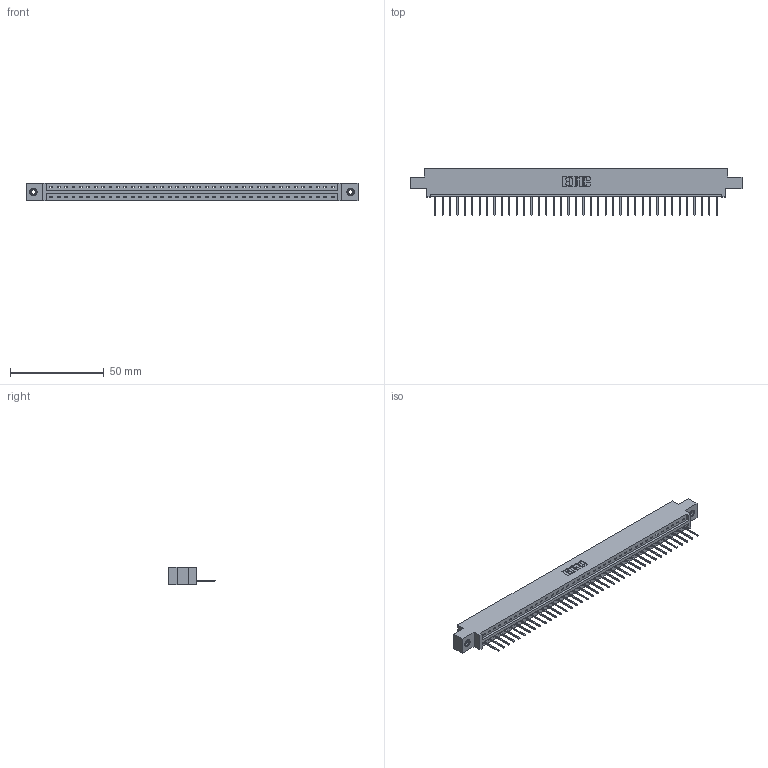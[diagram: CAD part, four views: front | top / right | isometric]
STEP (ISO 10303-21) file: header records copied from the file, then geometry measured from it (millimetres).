
FILE_DESCRIPTION (( 'STEP AP203' ), '1' );
FILE_NAME ('387-039-523-608.STEP', '2019-10-04T17:11:48', ( '' ), ( '' ), 'SwSTEP 2.0', 'SolidWorks 2016', '' );
FILE_SCHEMA (( 'CONFIG_CONTROL_DESIGN' ));
Length unit declared in the file: inch
Products named in the file (4): 337 Part_0.170 Offset - 0.156 Dia-TI; 345-250-001_345-250-003-102; 387-039-523-608; 345-292-001_345-293-123
Assembly tree (42 placements, depth 2):
  387-039-523-608
    337 Part_0.170 Offset - 0.156 Dia-TI
    345-292-001_345-293-123  x39
    345-250-001_345-250-003-102  x2
Bounding box: 177.55 x 25.15 x 9.4 mm (x, y, z)
Volume: 18276.3 mm3; surface area: 19029.7 mm2
Topology: 42 solids, 42 shells, 2596 faces, 7791 edges, 5134 vertices
Faces by surface type: plane 1900, cylinder 680, cone 12, torus 4
Entity records: 30714 total; most frequent: CARTESIAN_POINT 5330, ORIENTED_EDGE 5298, DIRECTION 4525, EDGE_CURVE 2649, LINE 2501, VECTOR 2501, VERTEX_POINT 1760, AXIS2_PLACEMENT_3D 1012
